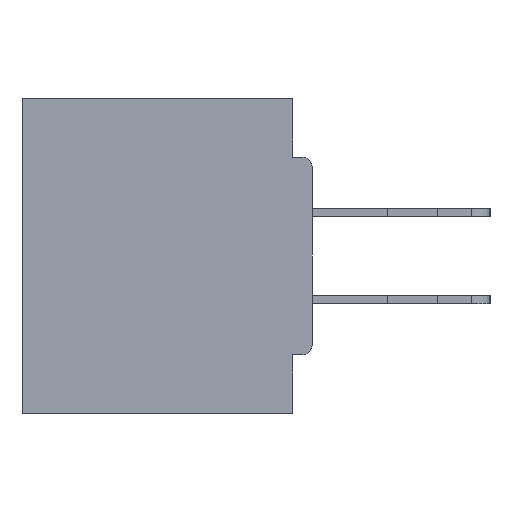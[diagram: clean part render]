
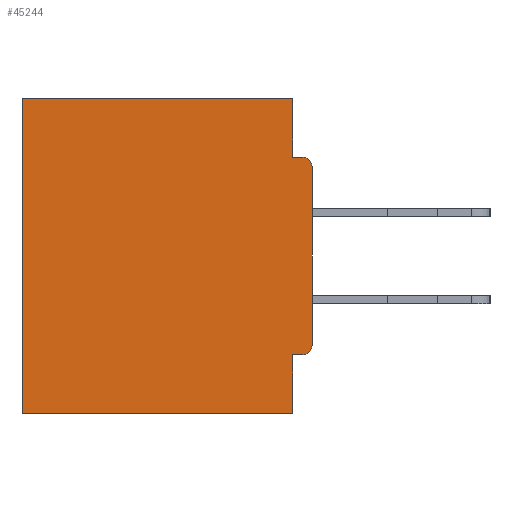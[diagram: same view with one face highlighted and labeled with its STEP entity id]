
A CAD part, left-side view. The second image highlights one B-rep face of the part: STEP entity #45244.
In plain terms, the highlighted planar face has unit normal (-1, 0, 0).
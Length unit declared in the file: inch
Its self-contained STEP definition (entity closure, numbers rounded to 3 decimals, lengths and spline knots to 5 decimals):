
#564 = ORIENTED_EDGE ( 'NONE', *, *, #12054, .F. ) ;
#1451 = DIRECTION ( 'NONE',  ( 0., 1., 0. ) ) ;
#2298 = LINE ( 'NONE', #2536, #16254 ) ;
#2336 = CARTESIAN_POINT ( 'NONE',  ( 0.298, 0., 0. ) ) ;
#2536 = CARTESIAN_POINT ( 'NONE',  ( 0.298, 0., 0. ) ) ;
#2798 = ORIENTED_EDGE ( 'NONE', *, *, #39185, .F. ) ;
#4062 = LINE ( 'NONE', #28299, #21920 ) ;
#4467 = VECTOR ( 'NONE', #5844, 39.37008 ) ;
#5223 = CARTESIAN_POINT ( 'NONE',  ( 0.298, 0., -0.5 ) ) ;
#5392 = ORIENTED_EDGE ( 'NONE', *, *, #16795, .F. ) ;
#5844 = DIRECTION ( 'NONE',  ( 0., 0., -1. ) ) ;
#6258 = DIRECTION ( 'NONE',  ( 1., 0., 0. ) ) ;
#6459 = AXIS2_PLACEMENT_3D ( 'NONE', #18257, #35854, #14054 ) ;
#6743 = VECTOR ( 'NONE', #1451, 39.37008 ) ;
#7744 = FACE_OUTER_BOUND ( 'NONE', #13308, .T. ) ;
#7818 = VERTEX_POINT ( 'NONE', #31288 ) ;
#7819 = CARTESIAN_POINT ( 'NONE',  ( 0.298, 0., -0.3915 ) ) ;
#8300 = DIRECTION ( 'NONE',  ( 0., -1., 0. ) ) ;
#8411 = VERTEX_POINT ( 'NONE', #9823 ) ;
#8559 = DIRECTION ( 'NONE',  ( 0., 0., -1. ) ) ;
#8749 = EDGE_CURVE ( 'NONE', #16072, #23950, #15317, .T. ) ;
#8901 = LINE ( 'NONE', #23902, #4467 ) ;
#9176 = DIRECTION ( 'NONE',  ( 0., 0., -1. ) ) ;
#9179 = CARTESIAN_POINT ( 'NONE',  ( 0.298, 0.031, -0.5 ) ) ;
#9548 = DIRECTION ( 'NONE',  ( 0., 1., 0. ) ) ;
#9823 = CARTESIAN_POINT ( 'NONE',  ( 0.298, 0.46, -0.5 ) ) ;
#11543 = DIRECTION ( 'NONE',  ( 0., 1., 0. ) ) ;
#11862 = VECTOR ( 'NONE', #31749, 39.37008 ) ;
#12054 = EDGE_CURVE ( 'NONE', #16669, #26712, #28812, .T. ) ;
#12962 = PLANE ( 'NONE',  #28992 ) ;
#13308 = EDGE_LOOP ( 'NONE', ( #32004, #564, #34505, #45773, #13790, #37194, #26832, #2798, #23479, #5392 ) ) ;
#13561 = CARTESIAN_POINT ( 'NONE',  ( 0.298, 0.031, -0.0935 ) ) ;
#13790 = ORIENTED_EDGE ( 'NONE', *, *, #28708, .T. ) ;
#14054 = DIRECTION ( 'NONE',  ( 0., 0., -1. ) ) ;
#14627 = LINE ( 'NONE', #45945, #11862 ) ;
#15273 = CARTESIAN_POINT ( 'NONE',  ( 0.298, 0.031, 0. ) ) ;
#15317 = CIRCLE ( 'NONE', #6459, 0.015 ) ;
#16072 = VERTEX_POINT ( 'NONE', #40329 ) ;
#16254 = VECTOR ( 'NONE', #9548, 39.37008 ) ;
#16350 = CIRCLE ( 'NONE', #45713, 0.015 ) ;
#16669 = VERTEX_POINT ( 'NONE', #13561 ) ;
#16795 = EDGE_CURVE ( 'NONE', #24383, #23950, #14627, .T. ) ;
#18257 = CARTESIAN_POINT ( 'NONE',  ( 0.298, 0.015, -0.3915 ) ) ;
#18929 = CARTESIAN_POINT ( 'NONE',  ( 0.298, 0., -0.0935 ) ) ;
#21000 = VECTOR ( 'NONE', #8300, 39.37008 ) ;
#21500 = EDGE_CURVE ( 'NONE', #24383, #26712, #16350, .T. ) ;
#21920 = VECTOR ( 'NONE', #45733, 39.37008 ) ;
#22008 = CARTESIAN_POINT ( 'NONE',  ( 0.298, 0., -0.4065 ) ) ;
#22334 = LINE ( 'NONE', #22008, #27899 ) ;
#23479 = ORIENTED_EDGE ( 'NONE', *, *, #8749, .T. ) ;
#23491 = LINE ( 'NONE', #5223, #6743 ) ;
#23508 = EDGE_CURVE ( 'NONE', #42833, #7818, #32346, .T. ) ;
#23902 = CARTESIAN_POINT ( 'NONE',  ( 0.298, 0.46, 0. ) ) ;
#23950 = VERTEX_POINT ( 'NONE', #7819 ) ;
#24383 = VERTEX_POINT ( 'NONE', #36895 ) ;
#26712 = VERTEX_POINT ( 'NONE', #33580 ) ;
#26832 = ORIENTED_EDGE ( 'NONE', *, *, #23508, .F. ) ;
#27899 = VECTOR ( 'NONE', #11543, 39.37008 ) ;
#28299 = CARTESIAN_POINT ( 'NONE',  ( 0.298, 0.031, -0.5 ) ) ;
#28563 = VERTEX_POINT ( 'NONE', #15273 ) ;
#28708 = EDGE_CURVE ( 'NONE', #31151, #8411, #8901, .T. ) ;
#28812 = LINE ( 'NONE', #18929, #21000 ) ;
#28992 = AXIS2_PLACEMENT_3D ( 'NONE', #2336, #6258, #44864 ) ;
#31151 = VERTEX_POINT ( 'NONE', #45632 ) ;
#31288 = CARTESIAN_POINT ( 'NONE',  ( 0.298, 0.031, -0.5 ) ) ;
#31749 = DIRECTION ( 'NONE',  ( 0., 0., -1. ) ) ;
#32004 = ORIENTED_EDGE ( 'NONE', *, *, #21500, .T. ) ;
#32346 = LINE ( 'NONE', #9179, #42946 ) ;
#32635 = EDGE_CURVE ( 'NONE', #28563, #16669, #4062, .T. ) ;
#33580 = CARTESIAN_POINT ( 'NONE',  ( 0.298, 0.015, -0.0935 ) ) ;
#33638 = CARTESIAN_POINT ( 'NONE',  ( 0.298, 0.015, -0.1085 ) ) ;
#34505 = ORIENTED_EDGE ( 'NONE', *, *, #32635, .F. ) ;
#35854 = DIRECTION ( 'NONE',  ( -1., 0., 0. ) ) ;
#36895 = CARTESIAN_POINT ( 'NONE',  ( 0.298, 0., -0.1085 ) ) ;
#37194 = ORIENTED_EDGE ( 'NONE', *, *, #38780, .F. ) ;
#37790 = CARTESIAN_POINT ( 'NONE',  ( 0.298, 0.031, -0.4065 ) ) ;
#38558 = EDGE_CURVE ( 'NONE', #28563, #31151, #2298, .T. ) ;
#38780 = EDGE_CURVE ( 'NONE', #7818, #8411, #23491, .T. ) ;
#39185 = EDGE_CURVE ( 'NONE', #16072, #42833, #22334, .T. ) ;
#40329 = CARTESIAN_POINT ( 'NONE',  ( 0.298, 0.015, -0.4065 ) ) ;
#40818 = DIRECTION ( 'NONE',  ( -1., 0., 0. ) ) ;
#42833 = VERTEX_POINT ( 'NONE', #37790 ) ;
#42946 = VECTOR ( 'NONE', #8559, 39.37008 ) ;
#44864 = DIRECTION ( 'NONE',  ( 0., 0., -1. ) ) ;
#45244 = ADVANCED_FACE ( 'NONE', ( #7744 ), #12962, .F. ) ;
#45632 = CARTESIAN_POINT ( 'NONE',  ( 0.298, 0.46, 0. ) ) ;
#45713 = AXIS2_PLACEMENT_3D ( 'NONE', #33638, #40818, #9176 ) ;
#45733 = DIRECTION ( 'NONE',  ( 0., 0., -1. ) ) ;
#45773 = ORIENTED_EDGE ( 'NONE', *, *, #38558, .T. ) ;
#45945 = CARTESIAN_POINT ( 'NONE',  ( 0.298, 0., 0. ) ) ;
